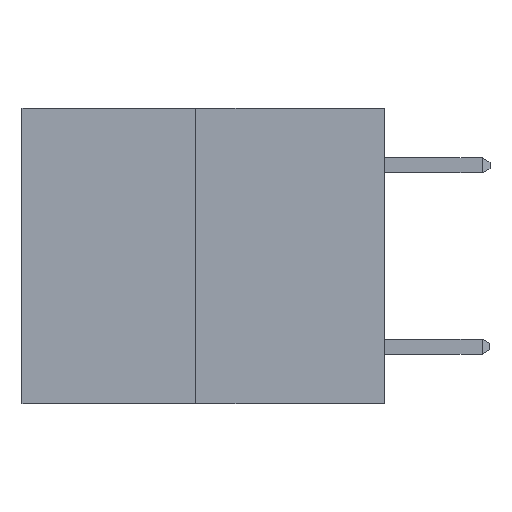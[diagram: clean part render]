
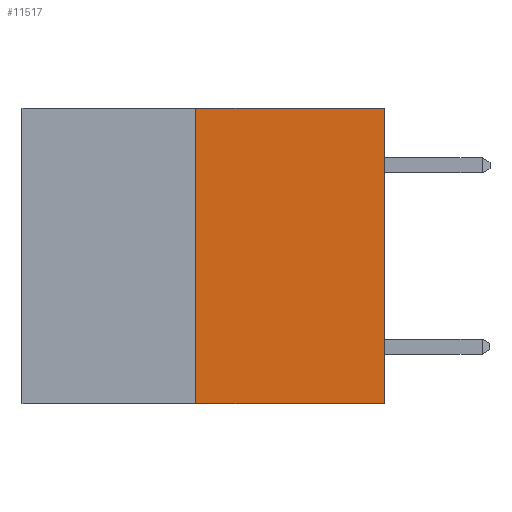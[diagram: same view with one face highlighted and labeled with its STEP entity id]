
A CAD part, left-side view. The second image highlights one B-rep face of the part: STEP entity #11517.
In plain terms, the highlighted planar face has unit normal (-1, 0, 0).
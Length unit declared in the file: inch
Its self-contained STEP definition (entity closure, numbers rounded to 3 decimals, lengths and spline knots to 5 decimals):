
#93 = VERTEX_POINT ( 'NONE', #10193 ) ;
#1575 = DIRECTION ( 'NONE',  ( 0., -1., 0. ) ) ;
#2070 = CARTESIAN_POINT ( 'NONE',  ( 0., 0.312, -0.49 ) ) ;
#2168 = ORIENTED_EDGE ( 'NONE', *, *, #18084, .F. ) ;
#2452 = CARTESIAN_POINT ( 'NONE',  ( 0., 0., 0. ) ) ;
#3373 = DIRECTION ( 'NONE',  ( 0., -1., 0. ) ) ;
#3511 = VECTOR ( 'NONE', #1575, 39.37008 ) ;
#3717 = ORIENTED_EDGE ( 'NONE', *, *, #16817, .T. ) ;
#4054 = DIRECTION ( 'NONE',  ( 0., 0., 1. ) ) ;
#4086 = DIRECTION ( 'NONE',  ( 1., 0., 0. ) ) ;
#6060 = EDGE_LOOP ( 'NONE', ( #2168, #3717, #15100, #7788 ) ) ;
#6631 = LINE ( 'NONE', #8830, #19845 ) ;
#6696 = CARTESIAN_POINT ( 'NONE',  ( 0., 0., 0. ) ) ;
#7253 = DIRECTION ( 'NONE',  ( 0., 0., -1. ) ) ;
#7700 = FACE_OUTER_BOUND ( 'NONE', #6060, .T. ) ;
#7788 = ORIENTED_EDGE ( 'NONE', *, *, #8902, .F. ) ;
#8818 = VERTEX_POINT ( 'NONE', #6696 ) ;
#8830 = CARTESIAN_POINT ( 'NONE',  ( 0., 0.312, -0.49 ) ) ;
#8902 = EDGE_CURVE ( 'NONE', #93, #8818, #14567, .T. ) ;
#9537 = VERTEX_POINT ( 'NONE', #2070 ) ;
#10193 = CARTESIAN_POINT ( 'NONE',  ( 0., 0.312, 0. ) ) ;
#11517 = ADVANCED_FACE ( 'NONE', ( #7700 ), #13562, .F. ) ;
#13377 = LINE ( 'NONE', #19628, #3511 ) ;
#13562 = PLANE ( 'NONE',  #13955 ) ;
#13638 = EDGE_CURVE ( 'NONE', #14862, #8818, #20929, .T. ) ;
#13955 = AXIS2_PLACEMENT_3D ( 'NONE', #15224, #4086, #7253 ) ;
#14567 = LINE ( 'NONE', #17894, #18200 ) ;
#14862 = VERTEX_POINT ( 'NONE', #18026 ) ;
#15052 = VECTOR ( 'NONE', #4054, 39.37008 ) ;
#15100 = ORIENTED_EDGE ( 'NONE', *, *, #13638, .T. ) ;
#15224 = CARTESIAN_POINT ( 'NONE',  ( 0., 0.6, 0. ) ) ;
#15377 = DIRECTION ( 'NONE',  ( 0., 0., 1. ) ) ;
#16817 = EDGE_CURVE ( 'NONE', #9537, #14862, #13377, .T. ) ;
#17894 = CARTESIAN_POINT ( 'NONE',  ( 0., 0.6, 0. ) ) ;
#18026 = CARTESIAN_POINT ( 'NONE',  ( 0., 0., -0.49 ) ) ;
#18084 = EDGE_CURVE ( 'NONE', #9537, #93, #6631, .T. ) ;
#18200 = VECTOR ( 'NONE', #3373, 39.37008 ) ;
#19628 = CARTESIAN_POINT ( 'NONE',  ( 0., 0.6, -0.49 ) ) ;
#19845 = VECTOR ( 'NONE', #15377, 39.37008 ) ;
#20929 = LINE ( 'NONE', #2452, #15052 ) ;
